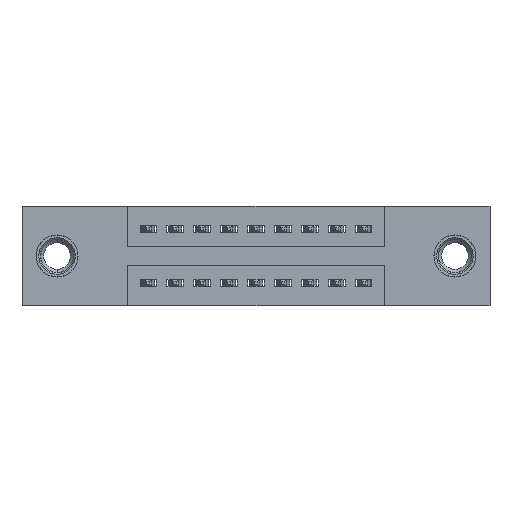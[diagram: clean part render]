
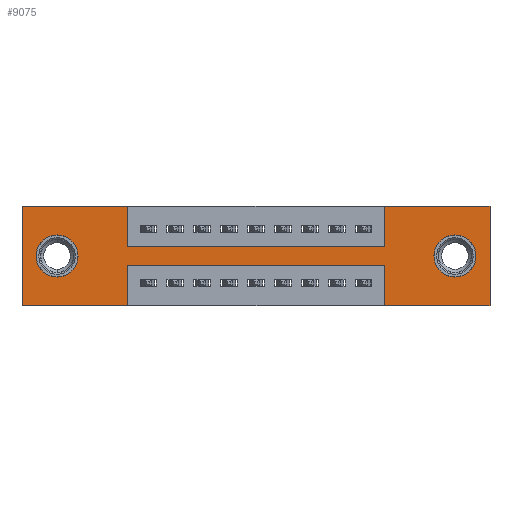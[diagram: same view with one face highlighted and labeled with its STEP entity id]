
A CAD part, front view. The second image highlights one B-rep face of the part: STEP entity #9075.
In plain terms, the highlighted planar face has unit normal (0, -1, 0).
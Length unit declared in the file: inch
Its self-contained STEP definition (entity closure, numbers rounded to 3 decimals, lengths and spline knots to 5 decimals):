
#200 = CARTESIAN_POINT ( 'NONE',  ( 0.13, 0., -0.185 ) ) ;
#307 = VERTEX_POINT ( 'NONE', #10404 ) ;
#372 = CARTESIAN_POINT ( 'NONE',  ( 0., 0., 0. ) ) ;
#418 = DIRECTION ( 'NONE',  ( 0., 0., 1. ) ) ;
#449 = EDGE_CURVE ( 'NONE', #6362, #2531, #5859, .T. ) ;
#553 = VECTOR ( 'NONE', #12245, 39.37008 ) ;
#689 = ORIENTED_EDGE ( 'NONE', *, *, #6290, .F. ) ;
#722 = ORIENTED_EDGE ( 'NONE', *, *, #9749, .F. ) ;
#741 = ORIENTED_EDGE ( 'NONE', *, *, #7166, .F. ) ;
#790 = LINE ( 'NONE', #5978, #5480 ) ;
#828 = ORIENTED_EDGE ( 'NONE', *, *, #3610, .F. ) ;
#923 = ORIENTED_EDGE ( 'NONE', *, *, #11809, .F. ) ;
#1018 = VECTOR ( 'NONE', #10781, 39.37008 ) ;
#1019 = ORIENTED_EDGE ( 'NONE', *, *, #7718, .F. ) ;
#1030 = EDGE_CURVE ( 'NONE', #1437, #10014, #12655, .T. ) ;
#1037 = LINE ( 'NONE', #10630, #11155 ) ;
#1052 = VECTOR ( 'NONE', #10995, 39.37008 ) ;
#1120 = ORIENTED_EDGE ( 'NONE', *, *, #12210, .F. ) ;
#1218 = ORIENTED_EDGE ( 'NONE', *, *, #449, .F. ) ;
#1220 = DIRECTION ( 'NONE',  ( 0., 1., 0. ) ) ;
#1242 = ORIENTED_EDGE ( 'NONE', *, *, #1506, .F. ) ;
#1295 = ORIENTED_EDGE ( 'NONE', *, *, #6776, .F. ) ;
#1310 = ORIENTED_EDGE ( 'NONE', *, *, #2842, .F. ) ;
#1353 = ORIENTED_EDGE ( 'NONE', *, *, #3691, .F. ) ;
#1382 = VECTOR ( 'NONE', #12420, 39.37008 ) ;
#1437 = VERTEX_POINT ( 'NONE', #2843 ) ;
#1506 = EDGE_CURVE ( 'NONE', #2531, #5629, #4018, .T. ) ;
#1785 = PLANE ( 'NONE',  #3931 ) ;
#1870 = CARTESIAN_POINT ( 'NONE',  ( 0., 0., 0. ) ) ;
#2048 = CARTESIAN_POINT ( 'NONE',  ( 1.3425, 0., -0.37 ) ) ;
#2201 = CARTESIAN_POINT ( 'NONE',  ( 0., 0., 0. ) ) ;
#2286 = VECTOR ( 'NONE', #9613, 39.37008 ) ;
#2437 = CARTESIAN_POINT ( 'NONE',  ( 1.3425, 0., 0. ) ) ;
#2453 = DIRECTION ( 'NONE',  ( 0., 1., 0. ) ) ;
#2531 = VERTEX_POINT ( 'NONE', #8178 ) ;
#2579 = CARTESIAN_POINT ( 'NONE',  ( 0.13, 0., -0.185 ) ) ;
#2585 = ORIENTED_EDGE ( 'NONE', *, *, #4995, .T. ) ;
#2632 = ORIENTED_EDGE ( 'NONE', *, *, #8622, .T. ) ;
#2693 = DIRECTION ( 'NONE',  ( 1., 0., 0. ) ) ;
#2723 = VERTEX_POINT ( 'NONE', #2816 ) ;
#2731 = CARTESIAN_POINT ( 'NONE',  ( 1.605, 0., -0.107 ) ) ;
#2796 = CARTESIAN_POINT ( 'NONE',  ( 0., 0., -0.37 ) ) ;
#2816 = CARTESIAN_POINT ( 'NONE',  ( 1.3425, 0., -0.22 ) ) ;
#2842 = EDGE_CURVE ( 'NONE', #307, #8869, #6277, .T. ) ;
#2843 = CARTESIAN_POINT ( 'NONE',  ( 0.13, 0., -0.263 ) ) ;
#2879 = VERTEX_POINT ( 'NONE', #2731 ) ;
#2956 = CARTESIAN_POINT ( 'NONE',  ( 0.3925, 0., -0.22 ) ) ;
#3022 = DIRECTION ( 'NONE',  ( -1., 0., 0. ) ) ;
#3151 = CARTESIAN_POINT ( 'NONE',  ( 0.3925, 0., -0.37 ) ) ;
#3157 = VERTEX_POINT ( 'NONE', #8925 ) ;
#3365 = CARTESIAN_POINT ( 'NONE',  ( 0.13, 0., -0.107 ) ) ;
#3426 = LINE ( 'NONE', #3477, #8572 ) ;
#3477 = CARTESIAN_POINT ( 'NONE',  ( 1.3425, 0., 0. ) ) ;
#3539 = AXIS2_PLACEMENT_3D ( 'NONE', #2579, #9383, #3591 ) ;
#3591 = DIRECTION ( 'NONE',  ( 0., 0., 1. ) ) ;
#3610 = EDGE_CURVE ( 'NONE', #6950, #4387, #790, .T. ) ;
#3676 = VECTOR ( 'NONE', #2693, 39.37008 ) ;
#3691 = EDGE_CURVE ( 'NONE', #7433, #6362, #7438, .T. ) ;
#3699 = CARTESIAN_POINT ( 'NONE',  ( 0.3925, 0., -0.15 ) ) ;
#3886 = DIRECTION ( 'NONE',  ( 0., 0., -1. ) ) ;
#3931 = AXIS2_PLACEMENT_3D ( 'NONE', #2796, #10551, #4782 ) ;
#3962 = DIRECTION ( 'NONE',  ( -1., 0., 0. ) ) ;
#4018 = LINE ( 'NONE', #372, #4326 ) ;
#4034 = EDGE_LOOP ( 'NONE', ( #2585, #2632 ) ) ;
#4227 = CARTESIAN_POINT ( 'NONE',  ( 1.735, 0., 0. ) ) ;
#4326 = VECTOR ( 'NONE', #418, 39.37008 ) ;
#4387 = VERTEX_POINT ( 'NONE', #7127 ) ;
#4429 = LINE ( 'NONE', #2956, #9252 ) ;
#4448 = CARTESIAN_POINT ( 'NONE',  ( 1.3425, 0., -0.15 ) ) ;
#4460 = DIRECTION ( 'NONE',  ( 0., 0., 1. ) ) ;
#4600 = FACE_BOUND ( 'NONE', #8890, .T. ) ;
#4690 = CARTESIAN_POINT ( 'NONE',  ( 0., 0., 0. ) ) ;
#4782 = DIRECTION ( 'NONE',  ( 0., 0., -1. ) ) ;
#4851 = CIRCLE ( 'NONE', #3539, 0.078 ) ;
#4899 = FACE_OUTER_BOUND ( 'NONE', #7205, .T. ) ;
#4936 = LINE ( 'NONE', #1870, #2286 ) ;
#4995 = EDGE_CURVE ( 'NONE', #2879, #7252, #8909, .T. ) ;
#5480 = VECTOR ( 'NONE', #3022, 39.37008 ) ;
#5629 = VERTEX_POINT ( 'NONE', #2201 ) ;
#5704 = LINE ( 'NONE', #4227, #1052 ) ;
#5859 = LINE ( 'NONE', #11480, #553 ) ;
#5978 = CARTESIAN_POINT ( 'NONE',  ( 0., 0., -0.37 ) ) ;
#6277 = LINE ( 'NONE', #3699, #3676 ) ;
#6290 = EDGE_CURVE ( 'NONE', #10758, #3157, #6336, .T. ) ;
#6336 = LINE ( 'NONE', #4690, #1382 ) ;
#6362 = VERTEX_POINT ( 'NONE', #6713 ) ;
#6551 = AXIS2_PLACEMENT_3D ( 'NONE', #200, #11470, #9830 ) ;
#6713 = CARTESIAN_POINT ( 'NONE',  ( 0.3925, 0., -0.37 ) ) ;
#6776 = EDGE_CURVE ( 'NONE', #8869, #10758, #3426, .T. ) ;
#6950 = VERTEX_POINT ( 'NONE', #10477 ) ;
#7111 = CARTESIAN_POINT ( 'NONE',  ( 1.605, 0., -0.185 ) ) ;
#7125 = VECTOR ( 'NONE', #8037, 39.37008 ) ;
#7127 = CARTESIAN_POINT ( 'NONE',  ( 1.3425, 0., -0.37 ) ) ;
#7158 = FACE_BOUND ( 'NONE', #4034, .T. ) ;
#7166 = EDGE_CURVE ( 'NONE', #4387, #2723, #9155, .T. ) ;
#7205 = EDGE_LOOP ( 'NONE', ( #1353, #722, #741, #828, #923, #689, #1295, #1310, #1120, #1019, #1242, #1218 ) ) ;
#7252 = VERTEX_POINT ( 'NONE', #9963 ) ;
#7433 = VERTEX_POINT ( 'NONE', #12190 ) ;
#7438 = LINE ( 'NONE', #3151, #7125 ) ;
#7718 = EDGE_CURVE ( 'NONE', #5629, #12659, #4936, .T. ) ;
#8037 = DIRECTION ( 'NONE',  ( 0., 0., -1. ) ) ;
#8086 = ORIENTED_EDGE ( 'NONE', *, *, #1030, .T. ) ;
#8091 = DIRECTION ( 'NONE',  ( 0., 0., -1. ) ) ;
#8178 = CARTESIAN_POINT ( 'NONE',  ( 0., 0., -0.37 ) ) ;
#8301 = CARTESIAN_POINT ( 'NONE',  ( 1.605, 0., -0.185 ) ) ;
#8572 = VECTOR ( 'NONE', #4460, 39.37008 ) ;
#8622 = EDGE_CURVE ( 'NONE', #7252, #2879, #10641, .T. ) ;
#8822 = ORIENTED_EDGE ( 'NONE', *, *, #10832, .T. ) ;
#8869 = VERTEX_POINT ( 'NONE', #4448 ) ;
#8890 = EDGE_LOOP ( 'NONE', ( #8822, #8086 ) ) ;
#8909 = CIRCLE ( 'NONE', #12487, 0.078 ) ;
#8925 = CARTESIAN_POINT ( 'NONE',  ( 1.735, 0., 0. ) ) ;
#9075 = ADVANCED_FACE ( 'NONE', ( #7158, #4600, #4899 ), #1785, .T. ) ;
#9155 = LINE ( 'NONE', #2048, #1018 ) ;
#9252 = VECTOR ( 'NONE', #3962, 39.37008 ) ;
#9266 = DIRECTION ( 'NONE',  ( 0., 0., -1. ) ) ;
#9383 = DIRECTION ( 'NONE',  ( 0., 1., 0. ) ) ;
#9525 = CARTESIAN_POINT ( 'NONE',  ( 0.3925, 0., 0. ) ) ;
#9576 = AXIS2_PLACEMENT_3D ( 'NONE', #8301, #2453, #9266 ) ;
#9613 = DIRECTION ( 'NONE',  ( 1., 0., 0. ) ) ;
#9749 = EDGE_CURVE ( 'NONE', #2723, #7433, #4429, .T. ) ;
#9830 = DIRECTION ( 'NONE',  ( 0., 0., 1. ) ) ;
#9963 = CARTESIAN_POINT ( 'NONE',  ( 1.605, 0., -0.263 ) ) ;
#10014 = VERTEX_POINT ( 'NONE', #3365 ) ;
#10404 = CARTESIAN_POINT ( 'NONE',  ( 0.3925, 0., -0.15 ) ) ;
#10477 = CARTESIAN_POINT ( 'NONE',  ( 1.735, 0., -0.37 ) ) ;
#10551 = DIRECTION ( 'NONE',  ( 0., -1., 0. ) ) ;
#10630 = CARTESIAN_POINT ( 'NONE',  ( 0.3925, 0., 0. ) ) ;
#10641 = CIRCLE ( 'NONE', #9576, 0.078 ) ;
#10758 = VERTEX_POINT ( 'NONE', #2437 ) ;
#10781 = DIRECTION ( 'NONE',  ( 0., 0., 1. ) ) ;
#10832 = EDGE_CURVE ( 'NONE', #10014, #1437, #4851, .T. ) ;
#10995 = DIRECTION ( 'NONE',  ( 0., 0., -1. ) ) ;
#11155 = VECTOR ( 'NONE', #3886, 39.37008 ) ;
#11470 = DIRECTION ( 'NONE',  ( 0., 1., 0. ) ) ;
#11480 = CARTESIAN_POINT ( 'NONE',  ( 0., 0., -0.37 ) ) ;
#11809 = EDGE_CURVE ( 'NONE', #3157, #6950, #5704, .T. ) ;
#12190 = CARTESIAN_POINT ( 'NONE',  ( 0.3925, 0., -0.22 ) ) ;
#12210 = EDGE_CURVE ( 'NONE', #12659, #307, #1037, .T. ) ;
#12245 = DIRECTION ( 'NONE',  ( -1., 0., 0. ) ) ;
#12420 = DIRECTION ( 'NONE',  ( 1., 0., 0. ) ) ;
#12487 = AXIS2_PLACEMENT_3D ( 'NONE', #7111, #1220, #8091 ) ;
#12655 = CIRCLE ( 'NONE', #6551, 0.078 ) ;
#12659 = VERTEX_POINT ( 'NONE', #9525 ) ;
